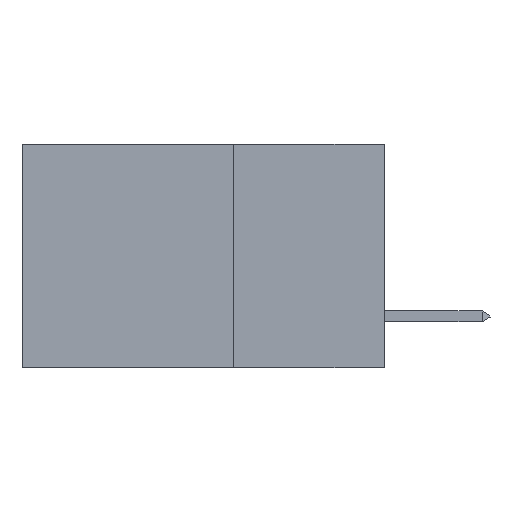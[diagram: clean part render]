
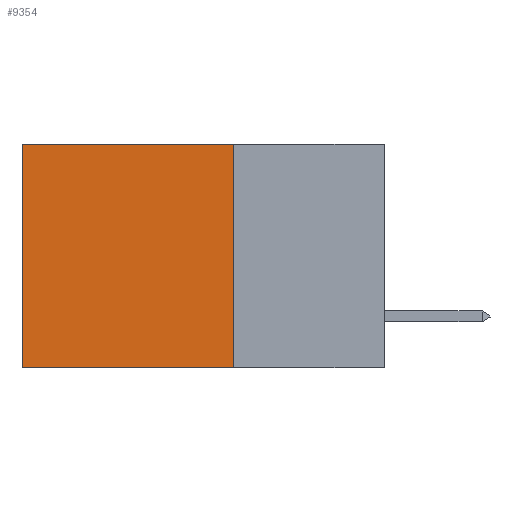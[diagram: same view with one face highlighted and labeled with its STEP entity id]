
A CAD part, left-side view. The second image highlights one B-rep face of the part: STEP entity #9354.
In plain terms, the highlighted planar face has unit normal (-1, 0, 0).
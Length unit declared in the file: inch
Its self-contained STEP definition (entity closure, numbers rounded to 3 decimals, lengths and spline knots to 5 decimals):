
#54 = ORIENTED_EDGE ( 'NONE', *, *, #14463, .F. ) ;
#388 = DIRECTION ( 'NONE',  ( 0., 0., -1. ) ) ;
#1049 = ORIENTED_EDGE ( 'NONE', *, *, #1255, .T. ) ;
#1092 = CARTESIAN_POINT ( 'NONE',  ( 0.2875, 0.25, -0.37 ) ) ;
#1248 = LINE ( 'NONE', #1092, #17968 ) ;
#1255 = EDGE_CURVE ( 'NONE', #22370, #12989, #22394, .T. ) ;
#2061 = CARTESIAN_POINT ( 'NONE',  ( 0.2875, 0.25, 0. ) ) ;
#4809 = AXIS2_PLACEMENT_3D ( 'NONE', #2061, #7506, #388 ) ;
#5271 = ORIENTED_EDGE ( 'NONE', *, *, #8850, .F. ) ;
#6439 = DIRECTION ( 'NONE',  ( 0., 1., 0. ) ) ;
#7308 = VECTOR ( 'NONE', #20407, 39.37008 ) ;
#7489 = VERTEX_POINT ( 'NONE', #16565 ) ;
#7506 = DIRECTION ( 'NONE',  ( 1., 0., 0. ) ) ;
#7594 = VECTOR ( 'NONE', #22109, 39.37008 ) ;
#8850 = EDGE_CURVE ( 'NONE', #22370, #7489, #9071, .T. ) ;
#9071 = LINE ( 'NONE', #22165, #11897 ) ;
#9354 = ADVANCED_FACE ( 'NONE', ( #18295 ), #11009, .F. ) ;
#10926 = CARTESIAN_POINT ( 'NONE',  ( 0.2875, 0.25, 0. ) ) ;
#11009 = PLANE ( 'NONE',  #4809 ) ;
#11897 = VECTOR ( 'NONE', #14907, 39.37008 ) ;
#12989 = VERTEX_POINT ( 'NONE', #16894 ) ;
#14463 = EDGE_CURVE ( 'NONE', #7489, #22389, #1248, .T. ) ;
#14907 = DIRECTION ( 'NONE',  ( 0., 0., -1. ) ) ;
#16534 = LINE ( 'NONE', #18598, #7308 ) ;
#16565 = CARTESIAN_POINT ( 'NONE',  ( 0.2875, 0.25, -0.37 ) ) ;
#16719 = EDGE_CURVE ( 'NONE', #12989, #22389, #16534, .T. ) ;
#16894 = CARTESIAN_POINT ( 'NONE',  ( 0.2875, 0.6, 0. ) ) ;
#17250 = CARTESIAN_POINT ( 'NONE',  ( 0.2875, 0.25, 0. ) ) ;
#17968 = VECTOR ( 'NONE', #6439, 39.37008 ) ;
#18295 = FACE_OUTER_BOUND ( 'NONE', #18852, .T. ) ;
#18598 = CARTESIAN_POINT ( 'NONE',  ( 0.2875, 0.6, 0. ) ) ;
#18852 = EDGE_LOOP ( 'NONE', ( #22418, #54, #5271, #1049 ) ) ;
#19617 = CARTESIAN_POINT ( 'NONE',  ( 0.2875, 0.6, -0.37 ) ) ;
#20407 = DIRECTION ( 'NONE',  ( 0., 0., -1. ) ) ;
#22109 = DIRECTION ( 'NONE',  ( 0., 1., 0. ) ) ;
#22165 = CARTESIAN_POINT ( 'NONE',  ( 0.2875, 0.25, 0. ) ) ;
#22370 = VERTEX_POINT ( 'NONE', #17250 ) ;
#22389 = VERTEX_POINT ( 'NONE', #19617 ) ;
#22394 = LINE ( 'NONE', #10926, #7594 ) ;
#22418 = ORIENTED_EDGE ( 'NONE', *, *, #16719, .T. ) ;
